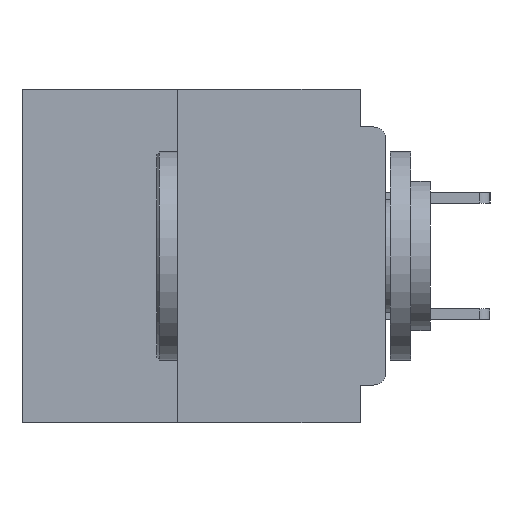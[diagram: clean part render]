
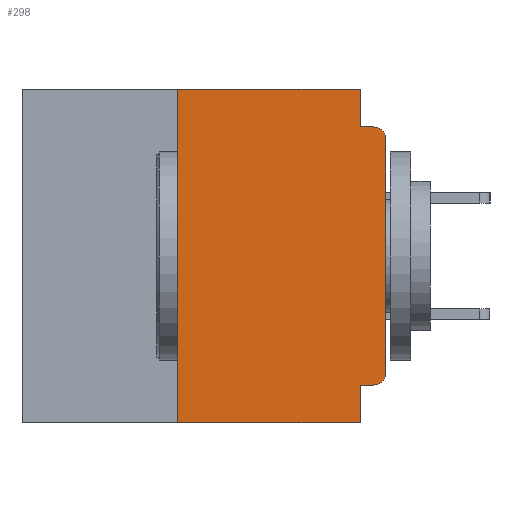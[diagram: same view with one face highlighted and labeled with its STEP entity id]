
A CAD part, left-side view. The second image highlights one B-rep face of the part: STEP entity #298.
In plain terms, the highlighted planar face has unit normal (-1, 0, 0).
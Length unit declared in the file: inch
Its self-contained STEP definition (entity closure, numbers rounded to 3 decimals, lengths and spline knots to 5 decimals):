
#298 = ADVANCED_FACE ( 'NONE', ( #14733 ), #1815, .F. ) ;
#875 = LINE ( 'NONE', #28516, #38895 ) ;
#1046 = DIRECTION ( 'NONE',  ( 0., 0., -1. ) ) ;
#1815 = PLANE ( 'NONE',  #29081 ) ;
#2349 = CARTESIAN_POINT ( 'NONE',  ( 0., 0., -0.355 ) ) ;
#2523 = DIRECTION ( 'NONE',  ( 0., 0., -1. ) ) ;
#2747 = DIRECTION ( 'NONE',  ( 0., -1., 0. ) ) ;
#2817 = DIRECTION ( 'NONE',  ( 1., 0., 0. ) ) ;
#3264 = ORIENTED_EDGE ( 'NONE', *, *, #41616, .F. ) ;
#3423 = VERTEX_POINT ( 'NONE', #10038 ) ;
#4665 = CARTESIAN_POINT ( 'NONE',  ( 0., 0., -0.06 ) ) ;
#4988 = EDGE_LOOP ( 'NONE', ( #27331, #19676, #58588, #13152, #3264, #47132, #28521, #39314, #37247, #49879 ) ) ;
#5363 = EDGE_CURVE ( 'NONE', #33005, #3423, #11087, .T. ) ;
#6148 = CARTESIAN_POINT ( 'NONE',  ( 0., 0.015, -0.045 ) ) ;
#6488 = EDGE_CURVE ( 'NONE', #53058, #41241, #56916, .T. ) ;
#6694 = VERTEX_POINT ( 'NONE', #29464 ) ;
#6988 = LINE ( 'NONE', #54428, #42116 ) ;
#7132 = VECTOR ( 'NONE', #54763, 39.37008 ) ;
#9546 = CARTESIAN_POINT ( 'NONE',  ( 0., 0.031, -0.4 ) ) ;
#9561 = AXIS2_PLACEMENT_3D ( 'NONE', #57405, #29984, #2523 ) ;
#10038 = CARTESIAN_POINT ( 'NONE',  ( 0., 0.031, -0.355 ) ) ;
#11087 = LINE ( 'NONE', #2349, #57773 ) ;
#11545 = CARTESIAN_POINT ( 'NONE',  ( 0., 0.031, -0.4 ) ) ;
#12194 = VERTEX_POINT ( 'NONE', #9546 ) ;
#13152 = ORIENTED_EDGE ( 'NONE', *, *, #24849, .F. ) ;
#13784 = EDGE_CURVE ( 'NONE', #33005, #6694, #18358, .T. ) ;
#14733 = FACE_OUTER_BOUND ( 'NONE', #4988, .T. ) ;
#15195 = LINE ( 'NONE', #57625, #25959 ) ;
#16020 = LINE ( 'NONE', #11545, #51128 ) ;
#16430 = LINE ( 'NONE', #59426, #7132 ) ;
#17737 = VECTOR ( 'NONE', #29797, 39.37008 ) ;
#17786 = DIRECTION ( 'NONE',  ( 0., -1., 0. ) ) ;
#18358 = CIRCLE ( 'NONE', #9561, 0.015 ) ;
#18426 = EDGE_CURVE ( 'NONE', #6694, #53058, #32189, .T. ) ;
#19676 = ORIENTED_EDGE ( 'NONE', *, *, #6488, .T. ) ;
#19830 = EDGE_CURVE ( 'NONE', #48594, #34418, #29958, .T. ) ;
#23865 = DIRECTION ( 'NONE',  ( -1., 0., 0. ) ) ;
#24405 = EDGE_CURVE ( 'NONE', #3423, #12194, #16020, .T. ) ;
#24849 = EDGE_CURVE ( 'NONE', #28982, #25998, #875, .T. ) ;
#25959 = VECTOR ( 'NONE', #2747, 39.37008 ) ;
#25998 = VERTEX_POINT ( 'NONE', #29714 ) ;
#26171 = CARTESIAN_POINT ( 'NONE',  ( 0., 0.437, 0. ) ) ;
#27331 = ORIENTED_EDGE ( 'NONE', *, *, #18426, .T. ) ;
#27426 = AXIS2_PLACEMENT_3D ( 'NONE', #51287, #23865, #55899 ) ;
#28516 = CARTESIAN_POINT ( 'NONE',  ( 0., 0.031, 0. ) ) ;
#28521 = ORIENTED_EDGE ( 'NONE', *, *, #32475, .T. ) ;
#28982 = VERTEX_POINT ( 'NONE', #50770 ) ;
#29081 = AXIS2_PLACEMENT_3D ( 'NONE', #26171, #2817, #39586 ) ;
#29464 = CARTESIAN_POINT ( 'NONE',  ( 0., 0., -0.34 ) ) ;
#29649 = CARTESIAN_POINT ( 'NONE',  ( 0., 0., 0. ) ) ;
#29714 = CARTESIAN_POINT ( 'NONE',  ( 0., 0.031, -0.045 ) ) ;
#29797 = DIRECTION ( 'NONE',  ( 0., 0., 1. ) ) ;
#29958 = LINE ( 'NONE', #34215, #17737 ) ;
#29984 = DIRECTION ( 'NONE',  ( -1., 0., 0. ) ) ;
#30751 = VECTOR ( 'NONE', #48060, 39.37008 ) ;
#32189 = LINE ( 'NONE', #29649, #30751 ) ;
#32475 = EDGE_CURVE ( 'NONE', #48594, #12194, #6988, .T. ) ;
#33005 = VERTEX_POINT ( 'NONE', #49792 ) ;
#34215 = CARTESIAN_POINT ( 'NONE',  ( 0., 0.25, -0.4 ) ) ;
#34418 = VERTEX_POINT ( 'NONE', #45817 ) ;
#37247 = ORIENTED_EDGE ( 'NONE', *, *, #5363, .F. ) ;
#38895 = VECTOR ( 'NONE', #1046, 39.37008 ) ;
#38972 = DIRECTION ( 'NONE',  ( 0., 0., -1. ) ) ;
#39003 = DIRECTION ( 'NONE',  ( 0., 1., 0. ) ) ;
#39314 = ORIENTED_EDGE ( 'NONE', *, *, #24405, .F. ) ;
#39586 = DIRECTION ( 'NONE',  ( 0., 0., -1. ) ) ;
#39665 = CARTESIAN_POINT ( 'NONE',  ( 0., 0.25, -0.4 ) ) ;
#41241 = VERTEX_POINT ( 'NONE', #6148 ) ;
#41616 = EDGE_CURVE ( 'NONE', #34418, #28982, #16430, .T. ) ;
#42116 = VECTOR ( 'NONE', #17786, 39.37008 ) ;
#45817 = CARTESIAN_POINT ( 'NONE',  ( 0., 0.25, 0. ) ) ;
#47132 = ORIENTED_EDGE ( 'NONE', *, *, #19830, .F. ) ;
#48060 = DIRECTION ( 'NONE',  ( 0., 0., 1. ) ) ;
#48594 = VERTEX_POINT ( 'NONE', #39665 ) ;
#49792 = CARTESIAN_POINT ( 'NONE',  ( 0., 0.015, -0.355 ) ) ;
#49879 = ORIENTED_EDGE ( 'NONE', *, *, #13784, .T. ) ;
#50770 = CARTESIAN_POINT ( 'NONE',  ( 0., 0.031, 0. ) ) ;
#51128 = VECTOR ( 'NONE', #38972, 39.37008 ) ;
#51287 = CARTESIAN_POINT ( 'NONE',  ( 0., 0.015, -0.06 ) ) ;
#53058 = VERTEX_POINT ( 'NONE', #4665 ) ;
#54428 = CARTESIAN_POINT ( 'NONE',  ( 0., 0.437, -0.4 ) ) ;
#54763 = DIRECTION ( 'NONE',  ( 0., -1., 0. ) ) ;
#55899 = DIRECTION ( 'NONE',  ( 0., 0., -1. ) ) ;
#56916 = CIRCLE ( 'NONE', #27426, 0.015 ) ;
#57405 = CARTESIAN_POINT ( 'NONE',  ( 0., 0.015, -0.34 ) ) ;
#57574 = EDGE_CURVE ( 'NONE', #25998, #41241, #15195, .T. ) ;
#57625 = CARTESIAN_POINT ( 'NONE',  ( 0., 0., -0.045 ) ) ;
#57773 = VECTOR ( 'NONE', #39003, 39.37008 ) ;
#58588 = ORIENTED_EDGE ( 'NONE', *, *, #57574, .F. ) ;
#59426 = CARTESIAN_POINT ( 'NONE',  ( 0., 0.437, 0. ) ) ;
